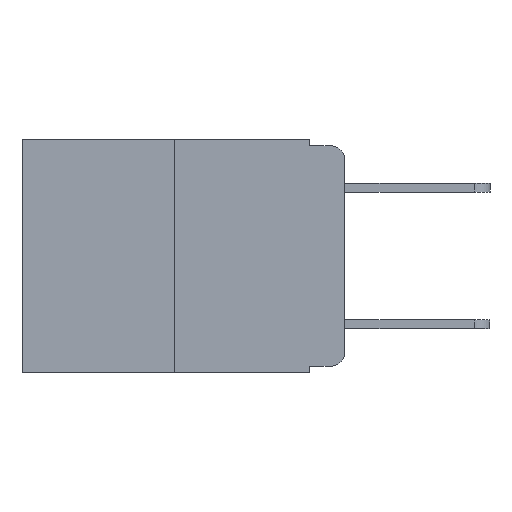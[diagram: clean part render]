
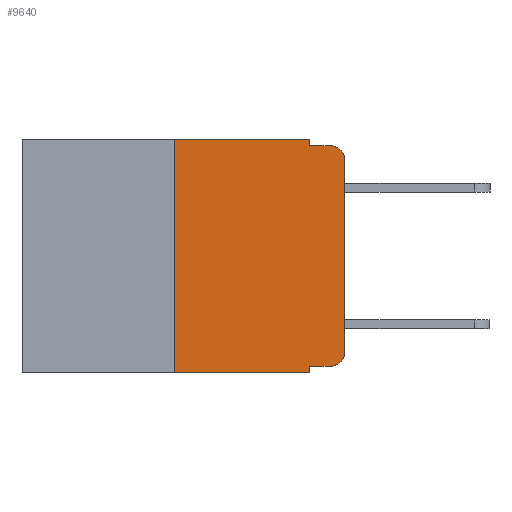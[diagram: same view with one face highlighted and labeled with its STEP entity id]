
A CAD part, left-side view. The second image highlights one B-rep face of the part: STEP entity #9640.
In plain terms, the highlighted planar face has unit normal (-1, 0, 0).
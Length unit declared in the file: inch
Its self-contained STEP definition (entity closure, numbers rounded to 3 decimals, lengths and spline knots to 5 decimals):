
#53 = CARTESIAN_POINT ( 'NONE',  ( 0., 0.051, -0.333 ) ) ;
#182 = CARTESIAN_POINT ( 'NONE',  ( 0., 0.473, 0. ) ) ;
#252 = EDGE_CURVE ( 'NONE', #17760, #14782, #22276, .T. ) ;
#582 = DIRECTION ( 'NONE',  ( -1., 0., 0. ) ) ;
#655 = EDGE_CURVE ( 'NONE', #20444, #19268, #5620, .T. ) ;
#738 = VERTEX_POINT ( 'NONE', #1631 ) ;
#893 = VERTEX_POINT ( 'NONE', #11950 ) ;
#946 = CIRCLE ( 'NONE', #15747, 0.02 ) ;
#947 = VECTOR ( 'NONE', #6317, 39.37008 ) ;
#1631 = CARTESIAN_POINT ( 'NONE',  ( 0., 0.051, 0. ) ) ;
#1696 = CARTESIAN_POINT ( 'NONE',  ( 0., 0.051, 0. ) ) ;
#1881 = CARTESIAN_POINT ( 'NONE',  ( 0., 0.25, -0.343 ) ) ;
#2397 = CARTESIAN_POINT ( 'NONE',  ( 0., 0., -0.313 ) ) ;
#2990 = CARTESIAN_POINT ( 'NONE',  ( 0., 0.051, -0.01 ) ) ;
#3247 = LINE ( 'NONE', #182, #16416 ) ;
#3447 = EDGE_CURVE ( 'NONE', #738, #20875, #21379, .T. ) ;
#3533 = DIRECTION ( 'NONE',  ( 0., 0., -1. ) ) ;
#3683 = ORIENTED_EDGE ( 'NONE', *, *, #655, .F. ) ;
#3837 = CARTESIAN_POINT ( 'NONE',  ( 0., 0.25, 0. ) ) ;
#4016 = LINE ( 'NONE', #7933, #21770 ) ;
#4078 = CARTESIAN_POINT ( 'NONE',  ( 0., 0.051, 0. ) ) ;
#4180 = PLANE ( 'NONE',  #13935 ) ;
#4381 = EDGE_CURVE ( 'NONE', #14543, #17760, #16690, .T. ) ;
#4649 = EDGE_CURVE ( 'NONE', #21865, #893, #13823, .T. ) ;
#5386 = DIRECTION ( 'NONE',  ( 0., 0., 1. ) ) ;
#5490 = CARTESIAN_POINT ( 'NONE',  ( 0., 0.051, -0.01 ) ) ;
#5620 = LINE ( 'NONE', #18902, #947 ) ;
#5945 = DIRECTION ( 'NONE',  ( 1., 0., 0. ) ) ;
#5957 = VECTOR ( 'NONE', #19024, 39.37008 ) ;
#6146 = ORIENTED_EDGE ( 'NONE', *, *, #9493, .F. ) ;
#6150 = CARTESIAN_POINT ( 'NONE',  ( 0., 0.02, -0.313 ) ) ;
#6206 = DIRECTION ( 'NONE',  ( -1., 0., 0. ) ) ;
#6317 = DIRECTION ( 'NONE',  ( 0., 0., 1. ) ) ;
#6498 = AXIS2_PLACEMENT_3D ( 'NONE', #6150, #6206, #6625 ) ;
#6625 = DIRECTION ( 'NONE',  ( 0., 0., -1. ) ) ;
#7571 = CARTESIAN_POINT ( 'NONE',  ( 0., 0.051, -0.333 ) ) ;
#7933 = CARTESIAN_POINT ( 'NONE',  ( 0., 0.473, -0.343 ) ) ;
#8190 = VECTOR ( 'NONE', #3533, 39.37008 ) ;
#8278 = VECTOR ( 'NONE', #19362, 39.37008 ) ;
#8806 = ORIENTED_EDGE ( 'NONE', *, *, #10159, .T. ) ;
#9493 = EDGE_CURVE ( 'NONE', #20875, #11298, #17457, .T. ) ;
#9562 = ORIENTED_EDGE ( 'NONE', *, *, #252, .T. ) ;
#9640 = ADVANCED_FACE ( 'NONE', ( #18836 ), #4180, .F. ) ;
#10159 = EDGE_CURVE ( 'NONE', #20444, #893, #4016, .T. ) ;
#10438 = DIRECTION ( 'NONE',  ( 0., -1., 0. ) ) ;
#10441 = LINE ( 'NONE', #53, #5957 ) ;
#10890 = CARTESIAN_POINT ( 'NONE',  ( 0., 0.02, -0.03 ) ) ;
#11298 = VERTEX_POINT ( 'NONE', #16544 ) ;
#11950 = CARTESIAN_POINT ( 'NONE',  ( 0., 0.051, -0.343 ) ) ;
#12149 = ORIENTED_EDGE ( 'NONE', *, *, #16943, .F. ) ;
#12526 = DIRECTION ( 'NONE',  ( 0., 0., -1. ) ) ;
#12747 = VECTOR ( 'NONE', #20961, 39.37008 ) ;
#13002 = CARTESIAN_POINT ( 'NONE',  ( 0., 0., -0.03 ) ) ;
#13235 = ORIENTED_EDGE ( 'NONE', *, *, #4649, .F. ) ;
#13270 = EDGE_CURVE ( 'NONE', #14782, #11298, #946, .T. ) ;
#13823 = LINE ( 'NONE', #1696, #8278 ) ;
#13935 = AXIS2_PLACEMENT_3D ( 'NONE', #19610, #5945, #17918 ) ;
#14371 = ORIENTED_EDGE ( 'NONE', *, *, #18169, .T. ) ;
#14543 = VERTEX_POINT ( 'NONE', #19415 ) ;
#14782 = VERTEX_POINT ( 'NONE', #13002 ) ;
#14925 = ORIENTED_EDGE ( 'NONE', *, *, #4381, .T. ) ;
#15731 = ORIENTED_EDGE ( 'NONE', *, *, #3447, .F. ) ;
#15747 = AXIS2_PLACEMENT_3D ( 'NONE', #10890, #582, #12526 ) ;
#16416 = VECTOR ( 'NONE', #10438, 39.37008 ) ;
#16544 = CARTESIAN_POINT ( 'NONE',  ( 0., 0.02, -0.01 ) ) ;
#16690 = CIRCLE ( 'NONE', #6498, 0.02 ) ;
#16943 = EDGE_CURVE ( 'NONE', #19268, #738, #3247, .T. ) ;
#17457 = LINE ( 'NONE', #5490, #12747 ) ;
#17685 = VECTOR ( 'NONE', #5386, 39.37008 ) ;
#17760 = VERTEX_POINT ( 'NONE', #2397 ) ;
#17918 = DIRECTION ( 'NONE',  ( 0., 0., -1. ) ) ;
#18169 = EDGE_CURVE ( 'NONE', #21865, #14543, #10441, .T. ) ;
#18836 = FACE_OUTER_BOUND ( 'NONE', #18886, .T. ) ;
#18886 = EDGE_LOOP ( 'NONE', ( #9562, #19291, #6146, #15731, #12149, #3683, #8806, #13235, #14371, #14925 ) ) ;
#18902 = CARTESIAN_POINT ( 'NONE',  ( 0., 0.25, 0. ) ) ;
#19024 = DIRECTION ( 'NONE',  ( 0., -1., 0. ) ) ;
#19268 = VERTEX_POINT ( 'NONE', #3837 ) ;
#19291 = ORIENTED_EDGE ( 'NONE', *, *, #13270, .T. ) ;
#19362 = DIRECTION ( 'NONE',  ( 0., 0., -1. ) ) ;
#19415 = CARTESIAN_POINT ( 'NONE',  ( 0., 0.02, -0.333 ) ) ;
#19610 = CARTESIAN_POINT ( 'NONE',  ( 0., 0.473, 0. ) ) ;
#20444 = VERTEX_POINT ( 'NONE', #1881 ) ;
#20847 = CARTESIAN_POINT ( 'NONE',  ( 0., 0., 0. ) ) ;
#20875 = VERTEX_POINT ( 'NONE', #2990 ) ;
#20961 = DIRECTION ( 'NONE',  ( 0., -1., 0. ) ) ;
#21379 = LINE ( 'NONE', #4078, #8190 ) ;
#21686 = DIRECTION ( 'NONE',  ( 0., -1., 0. ) ) ;
#21770 = VECTOR ( 'NONE', #21686, 39.37008 ) ;
#21865 = VERTEX_POINT ( 'NONE', #7571 ) ;
#22276 = LINE ( 'NONE', #20847, #17685 ) ;
